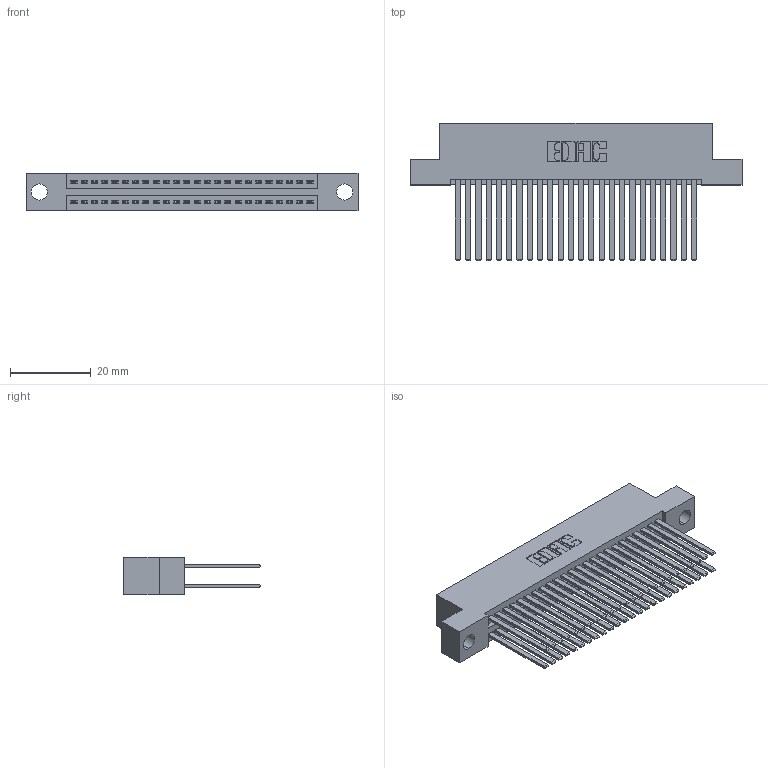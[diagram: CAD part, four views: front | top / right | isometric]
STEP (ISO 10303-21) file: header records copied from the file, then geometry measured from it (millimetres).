
FILE_DESCRIPTION (( 'STEP AP203' ), '1' );
FILE_NAME ('345-048-544-204.STEP', '2021-05-20T02:52:00', ( '' ), ( '' ), 'SwSTEP 2.0', 'SolidWorks 2020', '' );
FILE_SCHEMA (( 'CONFIG_CONTROL_DESIGN' ));
Length unit declared in the file: inch
Products named in the file (3): 345-048-544-204; 345 Part_Flush Mounting Lugs - 0.156 Dia-TI; 345-292-001_345-293-144
Assembly tree (49 placements, depth 2):
  345-048-544-204
    345 Part_Flush Mounting Lugs - 0.156 Dia-TI
    345-292-001_345-293-144  x48
Bounding box: 82.17 x 33.96 x 9.4 mm (x, y, z)
Volume: 8381.8 mm3; surface area: 13864.8 mm2
Topology: 49 solids, 49 shells, 2252 faces, 6665 edges, 4378 vertices
Faces by surface type: plane 1486, cylinder 766
Entity records: 21489 total; most frequent: CARTESIAN_POINT 3622, ORIENTED_EDGE 3554, DIRECTION 3213, EDGE_CURVE 1777, LINE 1553, VECTOR 1553, VERTEX_POINT 1182, AXIS2_PLACEMENT_3D 830
